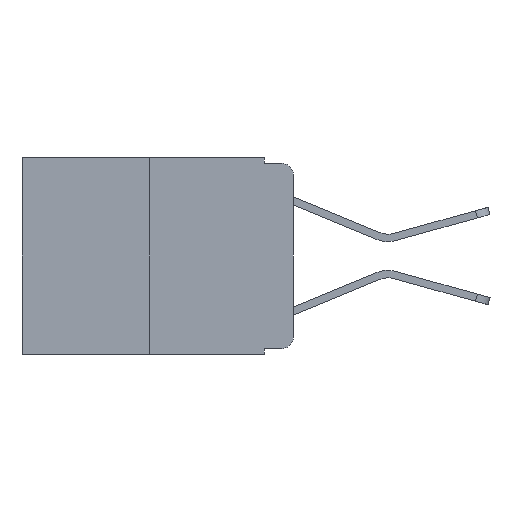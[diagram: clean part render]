
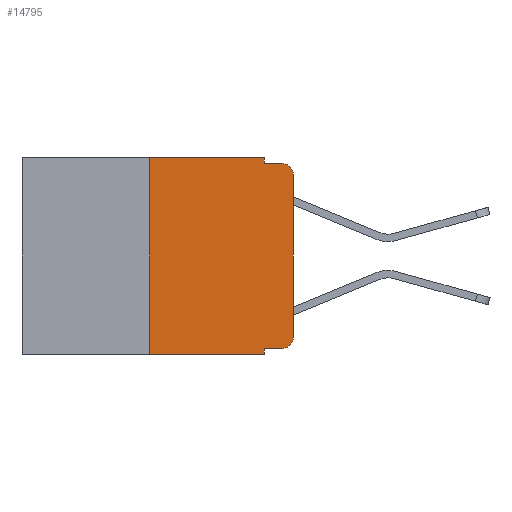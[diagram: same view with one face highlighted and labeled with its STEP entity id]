
A CAD part, left-side view. The second image highlights one B-rep face of the part: STEP entity #14795.
In plain terms, the highlighted planar face has unit normal (-1, 0, 0).
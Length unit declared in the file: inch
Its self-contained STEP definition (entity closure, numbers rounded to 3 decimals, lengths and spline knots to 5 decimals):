
#95 = ORIENTED_EDGE ( 'NONE', *, *, #6483, .T. ) ;
#347 = CARTESIAN_POINT ( 'NONE',  ( 0., 0.25, 0. ) ) ;
#478 = LINE ( 'NONE', #6146, #16100 ) ;
#530 = DIRECTION ( 'NONE',  ( 0., -1., 0. ) ) ;
#963 = ORIENTED_EDGE ( 'NONE', *, *, #16481, .F. ) ;
#1009 = CARTESIAN_POINT ( 'NONE',  ( 0., 0.25, -0.343 ) ) ;
#1051 = CARTESIAN_POINT ( 'NONE',  ( 0., 0.051, 0. ) ) ;
#1343 = DIRECTION ( 'NONE',  ( -1., 0., 0. ) ) ;
#1575 = DIRECTION ( 'NONE',  ( 0., 0., -1. ) ) ;
#2021 = VECTOR ( 'NONE', #14100, 39.37008 ) ;
#2316 = CARTESIAN_POINT ( 'NONE',  ( 0., 0.25, 0. ) ) ;
#2340 = CARTESIAN_POINT ( 'NONE',  ( 0., 0.473, 0. ) ) ;
#2499 = EDGE_CURVE ( 'NONE', #13299, #9752, #478, .T. ) ;
#2631 = CARTESIAN_POINT ( 'NONE',  ( 0., 0., -0.313 ) ) ;
#2752 = EDGE_CURVE ( 'NONE', #9752, #9612, #8544, .T. ) ;
#3502 = CARTESIAN_POINT ( 'NONE',  ( 0., 0.051, 0. ) ) ;
#4321 = CARTESIAN_POINT ( 'NONE',  ( 0., 0.02, -0.01 ) ) ;
#4838 = ORIENTED_EDGE ( 'NONE', *, *, #2499, .T. ) ;
#5091 = AXIS2_PLACEMENT_3D ( 'NONE', #2340, #9914, #12685 ) ;
#5222 = AXIS2_PLACEMENT_3D ( 'NONE', #15396, #1343, #8910 ) ;
#5396 = ORIENTED_EDGE ( 'NONE', *, *, #12515, .F. ) ;
#5631 = ORIENTED_EDGE ( 'NONE', *, *, #2752, .T. ) ;
#5682 = EDGE_CURVE ( 'NONE', #7241, #13299, #12645, .T. ) ;
#5777 = FACE_OUTER_BOUND ( 'NONE', #16148, .T. ) ;
#5910 = CARTESIAN_POINT ( 'NONE',  ( 0., 0.473, -0.343 ) ) ;
#6059 = ORIENTED_EDGE ( 'NONE', *, *, #9307, .F. ) ;
#6062 = LINE ( 'NONE', #8802, #13350 ) ;
#6146 = CARTESIAN_POINT ( 'NONE',  ( 0., 0., 0. ) ) ;
#6475 = CARTESIAN_POINT ( 'NONE',  ( 0., 0.051, -0.333 ) ) ;
#6483 = EDGE_CURVE ( 'NONE', #8799, #9902, #15880, .T. ) ;
#6700 = CARTESIAN_POINT ( 'NONE',  ( 0., 0.02, -0.03 ) ) ;
#7241 = VERTEX_POINT ( 'NONE', #14111 ) ;
#7265 = VERTEX_POINT ( 'NONE', #6475 ) ;
#7438 = VECTOR ( 'NONE', #15321, 39.37008 ) ;
#7587 = DIRECTION ( 'NONE',  ( -1., 0., 0. ) ) ;
#7750 = CARTESIAN_POINT ( 'NONE',  ( 0., 0.051, -0.333 ) ) ;
#8027 = ORIENTED_EDGE ( 'NONE', *, *, #5682, .T. ) ;
#8544 = CIRCLE ( 'NONE', #9900, 0.02 ) ;
#8713 = EDGE_CURVE ( 'NONE', #10306, #9612, #6062, .T. ) ;
#8799 = VERTEX_POINT ( 'NONE', #1009 ) ;
#8802 = CARTESIAN_POINT ( 'NONE',  ( 0., 0.051, -0.01 ) ) ;
#8910 = DIRECTION ( 'NONE',  ( 0., 0., -1. ) ) ;
#9307 = EDGE_CURVE ( 'NONE', #12277, #10306, #11311, .T. ) ;
#9355 = DIRECTION ( 'NONE',  ( 0., 0., 1. ) ) ;
#9612 = VERTEX_POINT ( 'NONE', #4321 ) ;
#9697 = LINE ( 'NONE', #3502, #2021 ) ;
#9752 = VERTEX_POINT ( 'NONE', #16585 ) ;
#9900 = AXIS2_PLACEMENT_3D ( 'NONE', #6700, #7587, #1575 ) ;
#9902 = VERTEX_POINT ( 'NONE', #14049 ) ;
#9904 = EDGE_CURVE ( 'NONE', #7265, #7241, #11843, .T. ) ;
#9914 = DIRECTION ( 'NONE',  ( 1., 0., 0. ) ) ;
#9966 = DIRECTION ( 'NONE',  ( 0., 0., 1. ) ) ;
#10149 = VECTOR ( 'NONE', #530, 39.37008 ) ;
#10216 = EDGE_CURVE ( 'NONE', #14046, #12277, #15702, .T. ) ;
#10306 = VERTEX_POINT ( 'NONE', #11150 ) ;
#10782 = DIRECTION ( 'NONE',  ( 0., -1., 0. ) ) ;
#10836 = ORIENTED_EDGE ( 'NONE', *, *, #8713, .F. ) ;
#10847 = CARTESIAN_POINT ( 'NONE',  ( 0., 0.473, 0. ) ) ;
#11150 = CARTESIAN_POINT ( 'NONE',  ( 0., 0.051, -0.01 ) ) ;
#11311 = LINE ( 'NONE', #1051, #7438 ) ;
#11623 = LINE ( 'NONE', #347, #13823 ) ;
#11843 = LINE ( 'NONE', #7750, #12038 ) ;
#12038 = VECTOR ( 'NONE', #12717, 39.37008 ) ;
#12265 = VECTOR ( 'NONE', #10782, 39.37008 ) ;
#12277 = VERTEX_POINT ( 'NONE', #13445 ) ;
#12515 = EDGE_CURVE ( 'NONE', #7265, #9902, #9697, .T. ) ;
#12587 = DIRECTION ( 'NONE',  ( 0., -1., 0. ) ) ;
#12645 = CIRCLE ( 'NONE', #5222, 0.02 ) ;
#12685 = DIRECTION ( 'NONE',  ( 0., 0., -1. ) ) ;
#12717 = DIRECTION ( 'NONE',  ( 0., -1., 0. ) ) ;
#13299 = VERTEX_POINT ( 'NONE', #2631 ) ;
#13350 = VECTOR ( 'NONE', #12587, 39.37008 ) ;
#13445 = CARTESIAN_POINT ( 'NONE',  ( 0., 0.051, 0. ) ) ;
#13589 = ORIENTED_EDGE ( 'NONE', *, *, #9904, .T. ) ;
#13823 = VECTOR ( 'NONE', #9355, 39.37008 ) ;
#13847 = ORIENTED_EDGE ( 'NONE', *, *, #10216, .F. ) ;
#14046 = VERTEX_POINT ( 'NONE', #2316 ) ;
#14049 = CARTESIAN_POINT ( 'NONE',  ( 0., 0.051, -0.343 ) ) ;
#14100 = DIRECTION ( 'NONE',  ( 0., 0., -1. ) ) ;
#14111 = CARTESIAN_POINT ( 'NONE',  ( 0., 0.02, -0.333 ) ) ;
#14795 = ADVANCED_FACE ( 'NONE', ( #5777 ), #16452, .F. ) ;
#15321 = DIRECTION ( 'NONE',  ( 0., 0., -1. ) ) ;
#15396 = CARTESIAN_POINT ( 'NONE',  ( 0., 0.02, -0.313 ) ) ;
#15702 = LINE ( 'NONE', #10847, #12265 ) ;
#15880 = LINE ( 'NONE', #5910, #10149 ) ;
#16100 = VECTOR ( 'NONE', #9966, 39.37008 ) ;
#16148 = EDGE_LOOP ( 'NONE', ( #4838, #5631, #10836, #6059, #13847, #963, #95, #5396, #13589, #8027 ) ) ;
#16452 = PLANE ( 'NONE',  #5091 ) ;
#16481 = EDGE_CURVE ( 'NONE', #8799, #14046, #11623, .T. ) ;
#16585 = CARTESIAN_POINT ( 'NONE',  ( 0., 0., -0.03 ) ) ;
